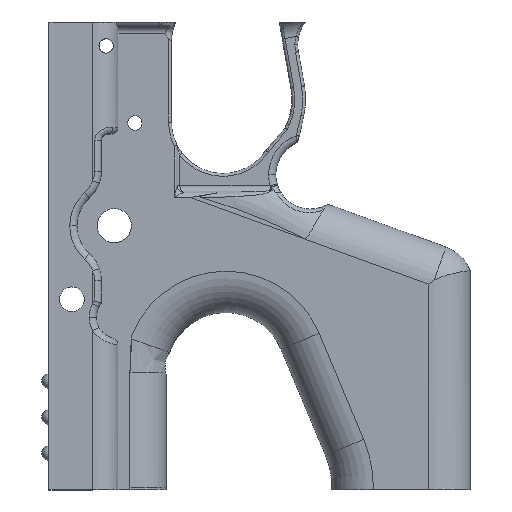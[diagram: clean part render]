
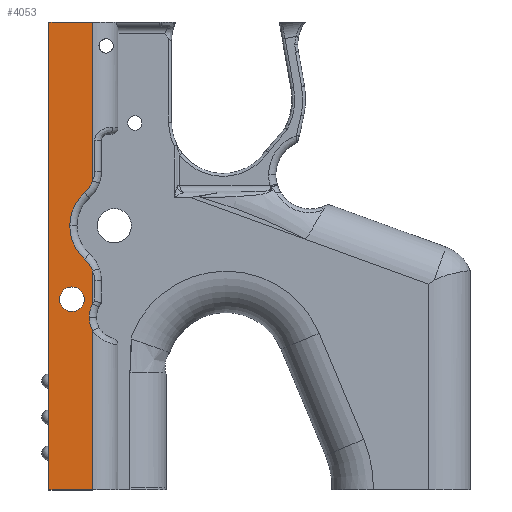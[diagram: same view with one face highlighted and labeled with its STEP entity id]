
A CAD part, left-side view. The second image highlights one B-rep face of the part: STEP entity #4053.
In plain terms, the highlighted planar face has unit normal (-1, 0, 0).
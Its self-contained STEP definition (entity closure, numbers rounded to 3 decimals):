
#133 = AXIS2_PLACEMENT_3D ( 'NONE', #1305, #2947, #9509 ) ;
#200 = CARTESIAN_POINT ( 'NONE',  ( -4.861, 21.06, 4.399 ) ) ;
#363 = CIRCLE ( 'NONE', #2193, 3.429 ) ;
#388 = DIRECTION ( 'NONE',  ( 1., 0., 0. ) ) ;
#475 = CIRCLE ( 'NONE', #3454, 8.01 ) ;
#489 = LINE ( 'NONE', #11656, #13890 ) ;
#1010 = CARTESIAN_POINT ( 'NONE',  ( -4.861, 27.406, 26.011 ) ) ;
#1105 = CARTESIAN_POINT ( 'NONE',  ( -4.861, 33.179, -47.364 ) ) ;
#1185 = EDGE_CURVE ( 'NONE', #3808, #7205, #6719, .T. ) ;
#1246 = EDGE_CURVE ( 'NONE', #3475, #3808, #5778, .T. ) ;
#1305 = CARTESIAN_POINT ( 'NONE',  ( -4.861, 14.002, 0.611 ) ) ;
#1345 = DIRECTION ( 'NONE',  ( 1., 0., 0. ) ) ;
#1443 = VERTEX_POINT ( 'NONE', #1010 ) ;
#1475 = CARTESIAN_POINT ( 'NONE',  ( -4.861, 21.06, 38.582 ) ) ;
#1516 = VECTOR ( 'NONE', #4124, 1000. ) ;
#1579 = ORIENTED_EDGE ( 'NONE', *, *, #12200, .T. ) ;
#1607 = EDGE_CURVE ( 'NONE', #2311, #8276, #475, .T. ) ;
#1901 = DIRECTION ( 'NONE',  ( 1., 0., 0. ) ) ;
#2008 = CARTESIAN_POINT ( 'NONE',  ( -4.861, 28.625, 41.182 ) ) ;
#2191 = AXIS2_PLACEMENT_3D ( 'NONE', #6375, #1901, #6151 ) ;
#2193 = AXIS2_PLACEMENT_3D ( 'NONE', #6734, #12018, #3282 ) ;
#2227 = ORIENTED_EDGE ( 'NONE', *, *, #5710, .F. ) ;
#2311 = VERTEX_POINT ( 'NONE', #7631 ) ;
#2360 = EDGE_LOOP ( 'NONE', ( #8063, #9011 ) ) ;
#2478 = CARTESIAN_POINT ( 'NONE',  ( -4.861, 21.06, 38.582 ) ) ;
#2539 = ORIENTED_EDGE ( 'NONE', *, *, #13075, .T. ) ;
#2675 = DIRECTION ( 'NONE',  ( -1., 0., 0. ) ) ;
#2704 = CARTESIAN_POINT ( 'NONE',  ( -4.861, 21.06, 4.399 ) ) ;
#2730 = VERTEX_POINT ( 'NONE', #11275 ) ;
#2786 = CARTESIAN_POINT ( 'NONE',  ( -4.861, 23.289, 35.222 ) ) ;
#2947 = DIRECTION ( 'NONE',  ( 1., 0., 0. ) ) ;
#2993 = ORIENTED_EDGE ( 'NONE', *, *, #1607, .T. ) ;
#3002 = EDGE_CURVE ( 'NONE', #14229, #3475, #8635, .T. ) ;
#3149 = EDGE_LOOP ( 'NONE', ( #13709, #1579, #12500, #12974, #5542, #12341, #2227, #2539, #2993, #9169, #9874, #6386 ) ) ;
#3282 = DIRECTION ( 'NONE',  ( 0., 0., 1. ) ) ;
#3344 = EDGE_CURVE ( 'NONE', #11881, #11684, #9565, .T. ) ;
#3454 = AXIS2_PLACEMENT_3D ( 'NONE', #12385, #1345, #4576 ) ;
#3475 = VERTEX_POINT ( 'NONE', #1475 ) ;
#3504 = FACE_OUTER_BOUND ( 'NONE', #3149, .T. ) ;
#3559 = CIRCLE ( 'NONE', #5397, 12.362 ) ;
#3808 = VERTEX_POINT ( 'NONE', #8353 ) ;
#3826 = CARTESIAN_POINT ( 'NONE',  ( -4.861, 28.625, 10.839 ) ) ;
#4014 = AXIS2_PLACEMENT_3D ( 'NONE', #3826, #2675, #11473 ) ;
#4053 = ADVANCED_FACE ( 'NONE', ( #3504, #7907 ), #7698, .T. ) ;
#4124 = DIRECTION ( 'NONE',  ( 0., 0., 1. ) ) ;
#4339 = LINE ( 'NONE', #8742, #1516 ) ;
#4377 = VECTOR ( 'NONE', #13441, 1000. ) ;
#4576 = DIRECTION ( 'NONE',  ( 0., 1., 0. ) ) ;
#4721 = AXIS2_PLACEMENT_3D ( 'NONE', #7886, #12229, #8973 ) ;
#5237 = EDGE_CURVE ( 'NONE', #8276, #7000, #10262, .T. ) ;
#5397 = AXIS2_PLACEMENT_3D ( 'NONE', #8305, #388, #8087 ) ;
#5523 = DIRECTION ( 'NONE',  ( -1., 0., 0. ) ) ;
#5542 = ORIENTED_EDGE ( 'NONE', *, *, #1185, .T. ) ;
#5610 = CARTESIAN_POINT ( 'NONE',  ( -4.861, 33.179, 82.636 ) ) ;
#5710 = EDGE_CURVE ( 'NONE', #2730, #6403, #12751, .T. ) ;
#5778 = LINE ( 'NONE', #2478, #4377 ) ;
#6097 = EDGE_CURVE ( 'NONE', #7000, #13912, #7015, .T. ) ;
#6151 = DIRECTION ( 'NONE',  ( 0., 1., 0. ) ) ;
#6375 = CARTESIAN_POINT ( 'NONE',  ( -4.861, 15.044, 26.011 ) ) ;
#6386 = ORIENTED_EDGE ( 'NONE', *, *, #11202, .T. ) ;
#6400 = DIRECTION ( 'NONE',  ( -1., 0., 0. ) ) ;
#6403 = VERTEX_POINT ( 'NONE', #1105 ) ;
#6719 = LINE ( 'NONE', #13165, #10598 ) ;
#6734 = CARTESIAN_POINT ( 'NONE',  ( -4.861, 26.817, 5.614 ) ) ;
#6994 = CARTESIAN_POINT ( 'NONE',  ( -4.861, 21.06, 13.44 ) ) ;
#7000 = VERTEX_POINT ( 'NONE', #200 ) ;
#7015 = LINE ( 'NONE', #2704, #10465 ) ;
#7205 = VERTEX_POINT ( 'NONE', #5610 ) ;
#7631 = CARTESIAN_POINT ( 'NONE',  ( -4.861, 21.06, -3.178 ) ) ;
#7657 = EDGE_CURVE ( 'NONE', #8162, #1443, #10482, .T. ) ;
#7698 = PLANE ( 'NONE',  #10499 ) ;
#7886 = CARTESIAN_POINT ( 'NONE',  ( -4.861, 26.817, 5.614 ) ) ;
#7907 = FACE_BOUND ( 'NONE', #2360, .T. ) ;
#8063 = ORIENTED_EDGE ( 'NONE', *, *, #3344, .F. ) ;
#8087 = DIRECTION ( 'NONE',  ( 0., 1., 0. ) ) ;
#8162 = VERTEX_POINT ( 'NONE', #12139 ) ;
#8276 = VERTEX_POINT ( 'NONE', #10736 ) ;
#8305 = CARTESIAN_POINT ( 'NONE',  ( -4.861, 15.044, 26.011 ) ) ;
#8353 = CARTESIAN_POINT ( 'NONE',  ( -4.861, 21.06, 82.636 ) ) ;
#8378 = CARTESIAN_POINT ( 'NONE',  ( -4.861, 30.246, 5.614 ) ) ;
#8635 = CIRCLE ( 'NONE', #10953, 8. ) ;
#8742 = CARTESIAN_POINT ( 'NONE',  ( -4.861, 21.06, -47.364 ) ) ;
#8819 = DIRECTION ( 'NONE',  ( 0., 1., 0. ) ) ;
#8973 = DIRECTION ( 'NONE',  ( 0., 0., 1. ) ) ;
#9011 = ORIENTED_EDGE ( 'NONE', *, *, #10184, .F. ) ;
#9124 = DIRECTION ( 'NONE',  ( 0., 0., 1. ) ) ;
#9169 = ORIENTED_EDGE ( 'NONE', *, *, #5237, .T. ) ;
#9509 = DIRECTION ( 'NONE',  ( 0., 1., 0. ) ) ;
#9565 = CIRCLE ( 'NONE', #4721, 3.429 ) ;
#9874 = ORIENTED_EDGE ( 'NONE', *, *, #6097, .T. ) ;
#10184 = EDGE_CURVE ( 'NONE', #11684, #11881, #363, .T. ) ;
#10262 = CIRCLE ( 'NONE', #133, 8.01 ) ;
#10445 = DIRECTION ( 'NONE',  ( 0., 1., 0. ) ) ;
#10465 = VECTOR ( 'NONE', #9124, 1000. ) ;
#10482 = CIRCLE ( 'NONE', #2191, 12.362 ) ;
#10499 = AXIS2_PLACEMENT_3D ( 'NONE', #12110, #5523, #11093 ) ;
#10598 = VECTOR ( 'NONE', #8819, 1000. ) ;
#10736 = CARTESIAN_POINT ( 'NONE',  ( -4.861, 22.012, 0.611 ) ) ;
#10953 = AXIS2_PLACEMENT_3D ( 'NONE', #2008, #6400, #11743 ) ;
#11093 = DIRECTION ( 'NONE',  ( 0., 0., 1. ) ) ;
#11202 = EDGE_CURVE ( 'NONE', #13912, #8162, #14164, .T. ) ;
#11275 = CARTESIAN_POINT ( 'NONE',  ( -4.861, 21.06, -47.364 ) ) ;
#11473 = DIRECTION ( 'NONE',  ( 0., 1., 0. ) ) ;
#11656 = CARTESIAN_POINT ( 'NONE',  ( -4.861, 33.179, 167.539 ) ) ;
#11684 = VERTEX_POINT ( 'NONE', #13232 ) ;
#11738 = CARTESIAN_POINT ( 'NONE',  ( -4.861, 0., -47.364 ) ) ;
#11743 = DIRECTION ( 'NONE',  ( 0., 1., 0. ) ) ;
#11881 = VERTEX_POINT ( 'NONE', #8378 ) ;
#12018 = DIRECTION ( 'NONE',  ( -1., 0., 0. ) ) ;
#12110 = CARTESIAN_POINT ( 'NONE',  ( -4.861, 21.06, 146.035 ) ) ;
#12139 = CARTESIAN_POINT ( 'NONE',  ( -4.861, 23.289, 16.8 ) ) ;
#12200 = EDGE_CURVE ( 'NONE', #1443, #14229, #3559, .T. ) ;
#12229 = DIRECTION ( 'NONE',  ( -1., 0., 0. ) ) ;
#12341 = ORIENTED_EDGE ( 'NONE', *, *, #14207, .F. ) ;
#12385 = CARTESIAN_POINT ( 'NONE',  ( -4.861, 14.002, 0.611 ) ) ;
#12500 = ORIENTED_EDGE ( 'NONE', *, *, #3002, .T. ) ;
#12751 = LINE ( 'NONE', #11738, #13037 ) ;
#12974 = ORIENTED_EDGE ( 'NONE', *, *, #1246, .T. ) ;
#13037 = VECTOR ( 'NONE', #10445, 1000. ) ;
#13075 = EDGE_CURVE ( 'NONE', #2730, #2311, #4339, .T. ) ;
#13165 = CARTESIAN_POINT ( 'NONE',  ( -4.861, 21.06, 82.636 ) ) ;
#13232 = CARTESIAN_POINT ( 'NONE',  ( -4.861, 23.388, 5.614 ) ) ;
#13441 = DIRECTION ( 'NONE',  ( 0., 0., 1. ) ) ;
#13678 = DIRECTION ( 'NONE',  ( 0., 0., 1. ) ) ;
#13709 = ORIENTED_EDGE ( 'NONE', *, *, #7657, .T. ) ;
#13890 = VECTOR ( 'NONE', #13678, 1000. ) ;
#13912 = VERTEX_POINT ( 'NONE', #6994 ) ;
#14164 = CIRCLE ( 'NONE', #4014, 8. ) ;
#14207 = EDGE_CURVE ( 'NONE', #6403, #7205, #489, .T. ) ;
#14229 = VERTEX_POINT ( 'NONE', #2786 ) ;
